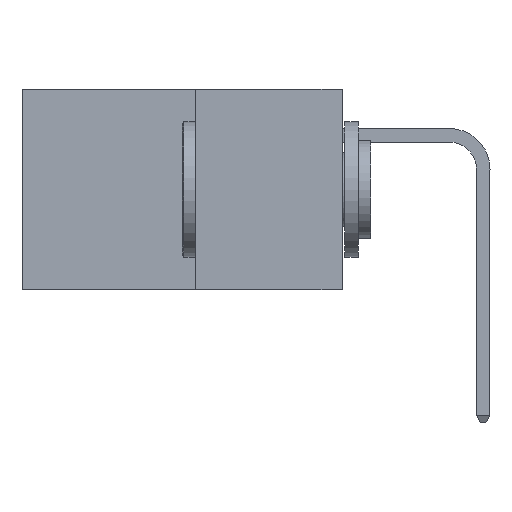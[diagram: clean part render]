
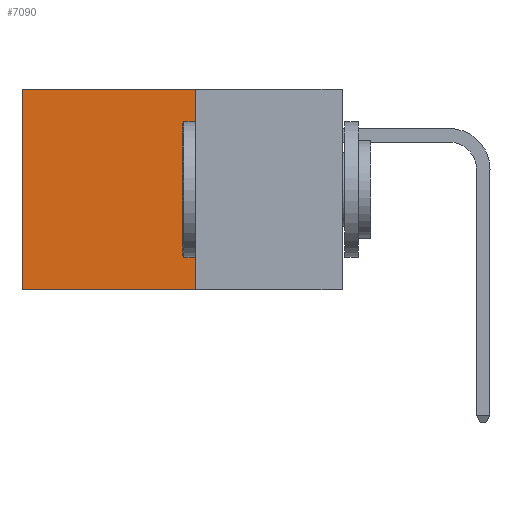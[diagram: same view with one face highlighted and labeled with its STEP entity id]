
A CAD part, left-side view. The second image highlights one B-rep face of the part: STEP entity #7090.
In plain terms, the highlighted planar face has unit normal (-1, 0, 0).
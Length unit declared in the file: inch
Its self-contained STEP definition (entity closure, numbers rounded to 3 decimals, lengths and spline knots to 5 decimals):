
#127 = CARTESIAN_POINT ( 'NONE',  ( 0.277, 0.59, -0.37 ) ) ;
#2483 = CARTESIAN_POINT ( 'NONE',  ( 0.277, 0.27, -0.37 ) ) ;
#2487 = DIRECTION ( 'NONE',  ( 0., 0., -1. ) ) ;
#2588 = LINE ( 'NONE', #127, #12672 ) ;
#2871 = CARTESIAN_POINT ( 'NONE',  ( 0.277, 0.27, 0. ) ) ;
#3211 = VERTEX_POINT ( 'NONE', #3883 ) ;
#3377 = ORIENTED_EDGE ( 'NONE', *, *, #19506, .T. ) ;
#3730 = VERTEX_POINT ( 'NONE', #11817 ) ;
#3883 = CARTESIAN_POINT ( 'NONE',  ( 0.277, 0.59, 0. ) ) ;
#4710 = EDGE_CURVE ( 'NONE', #13025, #12748, #14770, .T. ) ;
#4718 = ORIENTED_EDGE ( 'NONE', *, *, #6840, .F. ) ;
#4736 = VECTOR ( 'NONE', #9069, 39.37008 ) ;
#6504 = VECTOR ( 'NONE', #11548, 39.37008 ) ;
#6732 = CARTESIAN_POINT ( 'NONE',  ( 0.277, 0.27, -0.37 ) ) ;
#6840 = EDGE_CURVE ( 'NONE', #3730, #13025, #18695, .T. ) ;
#7090 = ADVANCED_FACE ( 'NONE', ( #13006 ), #17756, .F. ) ;
#7474 = ORIENTED_EDGE ( 'NONE', *, *, #14598, .T. ) ;
#9069 = DIRECTION ( 'NONE',  ( 0., 1., 0. ) ) ;
#9502 = ORIENTED_EDGE ( 'NONE', *, *, #4710, .F. ) ;
#11548 = DIRECTION ( 'NONE',  ( 0., 1., 0. ) ) ;
#11714 = CARTESIAN_POINT ( 'NONE',  ( 0.277, 0.27, -0.37 ) ) ;
#11817 = CARTESIAN_POINT ( 'NONE',  ( 0.277, 0.27, 0. ) ) ;
#12672 = VECTOR ( 'NONE', #15798, 39.37008 ) ;
#12748 = VERTEX_POINT ( 'NONE', #19885 ) ;
#13006 = FACE_OUTER_BOUND ( 'NONE', #18123, .T. ) ;
#13025 = VERTEX_POINT ( 'NONE', #6732 ) ;
#13193 = AXIS2_PLACEMENT_3D ( 'NONE', #17775, #17565, #17524 ) ;
#13532 = LINE ( 'NONE', #2871, #4736 ) ;
#13739 = VECTOR ( 'NONE', #2487, 39.37008 ) ;
#14598 = EDGE_CURVE ( 'NONE', #3730, #3211, #13532, .T. ) ;
#14770 = LINE ( 'NONE', #11714, #6504 ) ;
#15798 = DIRECTION ( 'NONE',  ( 0., 0., -1. ) ) ;
#17524 = DIRECTION ( 'NONE',  ( 0., 0., -1. ) ) ;
#17565 = DIRECTION ( 'NONE',  ( 1., 0., 0. ) ) ;
#17756 = PLANE ( 'NONE',  #13193 ) ;
#17775 = CARTESIAN_POINT ( 'NONE',  ( 0.277, 0.27, -0.37 ) ) ;
#18123 = EDGE_LOOP ( 'NONE', ( #3377, #9502, #4718, #7474 ) ) ;
#18695 = LINE ( 'NONE', #2483, #13739 ) ;
#19506 = EDGE_CURVE ( 'NONE', #3211, #12748, #2588, .T. ) ;
#19885 = CARTESIAN_POINT ( 'NONE',  ( 0.277, 0.59, -0.37 ) ) ;
